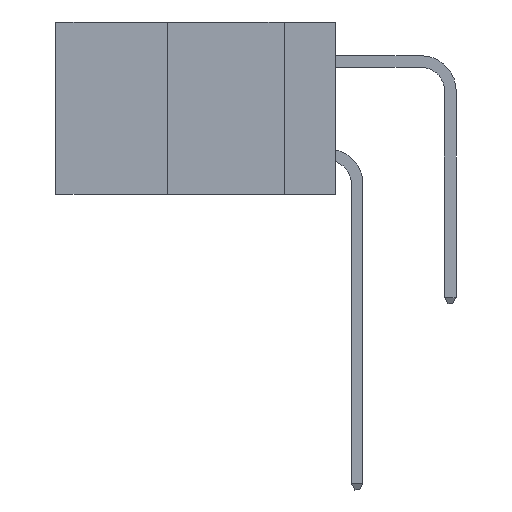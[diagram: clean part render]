
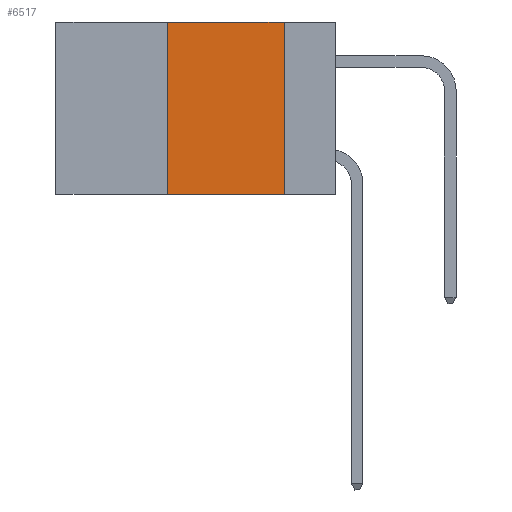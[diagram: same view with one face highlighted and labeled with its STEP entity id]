
A CAD part, left-side view. The second image highlights one B-rep face of the part: STEP entity #6517.
In plain terms, the highlighted planar face has unit normal (-1, 0, 0).
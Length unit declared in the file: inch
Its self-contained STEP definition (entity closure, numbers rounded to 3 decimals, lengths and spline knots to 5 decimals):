
#131 = ORIENTED_EDGE ( 'NONE', *, *, #6104, .F. ) ;
#926 = DIRECTION ( 'NONE',  ( 1., 0., 0. ) ) ;
#1832 = EDGE_LOOP ( 'NONE', ( #7850, #131, #11746, #3072 ) ) ;
#2141 = FACE_OUTER_BOUND ( 'NONE', #1832, .T. ) ;
#2537 = VERTEX_POINT ( 'NONE', #11503 ) ;
#2735 = VERTEX_POINT ( 'NONE', #10904 ) ;
#2875 = VERTEX_POINT ( 'NONE', #7464 ) ;
#3072 = ORIENTED_EDGE ( 'NONE', *, *, #9234, .T. ) ;
#3481 = CARTESIAN_POINT ( 'NONE',  ( 0., 0.11, -0.37 ) ) ;
#4071 = VECTOR ( 'NONE', #10566, 39.37008 ) ;
#4593 = DIRECTION ( 'NONE',  ( 0., -1., 0. ) ) ;
#5167 = CARTESIAN_POINT ( 'NONE',  ( 0., 0.6, -0.37 ) ) ;
#5271 = VECTOR ( 'NONE', #8865, 39.37008 ) ;
#5575 = LINE ( 'NONE', #11488, #5271 ) ;
#6104 = EDGE_CURVE ( 'NONE', #2875, #2537, #8981, .T. ) ;
#6131 = DIRECTION ( 'NONE',  ( 0., -1., 0. ) ) ;
#6517 = ADVANCED_FACE ( 'NONE', ( #2141 ), #12334, .F. ) ;
#7464 = CARTESIAN_POINT ( 'NONE',  ( 0., 0.36, 0. ) ) ;
#7850 = ORIENTED_EDGE ( 'NONE', *, *, #9988, .F. ) ;
#7915 = DIRECTION ( 'NONE',  ( 0., 0., -1. ) ) ;
#8177 = VECTOR ( 'NONE', #6131, 39.37008 ) ;
#8452 = LINE ( 'NONE', #5167, #8177 ) ;
#8685 = VECTOR ( 'NONE', #4593, 39.37008 ) ;
#8748 = LINE ( 'NONE', #8799, #4071 ) ;
#8776 = VERTEX_POINT ( 'NONE', #3481 ) ;
#8799 = CARTESIAN_POINT ( 'NONE',  ( 0., 0.36, 0. ) ) ;
#8865 = DIRECTION ( 'NONE',  ( 0., 0., -1. ) ) ;
#8981 = LINE ( 'NONE', #11823, #8685 ) ;
#9219 = EDGE_CURVE ( 'NONE', #2735, #2875, #8748, .T. ) ;
#9234 = EDGE_CURVE ( 'NONE', #2735, #8776, #8452, .T. ) ;
#9988 = EDGE_CURVE ( 'NONE', #2537, #8776, #5575, .T. ) ;
#10284 = AXIS2_PLACEMENT_3D ( 'NONE', #10569, #926, #7915 ) ;
#10566 = DIRECTION ( 'NONE',  ( 0., 0., 1. ) ) ;
#10569 = CARTESIAN_POINT ( 'NONE',  ( 0., 0.6, 0. ) ) ;
#10904 = CARTESIAN_POINT ( 'NONE',  ( 0., 0.36, -0.37 ) ) ;
#11488 = CARTESIAN_POINT ( 'NONE',  ( 0., 0.11, 0. ) ) ;
#11503 = CARTESIAN_POINT ( 'NONE',  ( 0., 0.11, 0. ) ) ;
#11746 = ORIENTED_EDGE ( 'NONE', *, *, #9219, .F. ) ;
#11823 = CARTESIAN_POINT ( 'NONE',  ( 0., 0.6, 0. ) ) ;
#12334 = PLANE ( 'NONE',  #10284 ) ;
